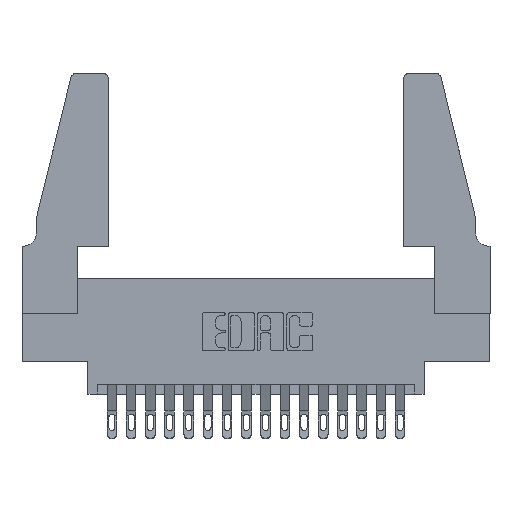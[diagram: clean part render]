
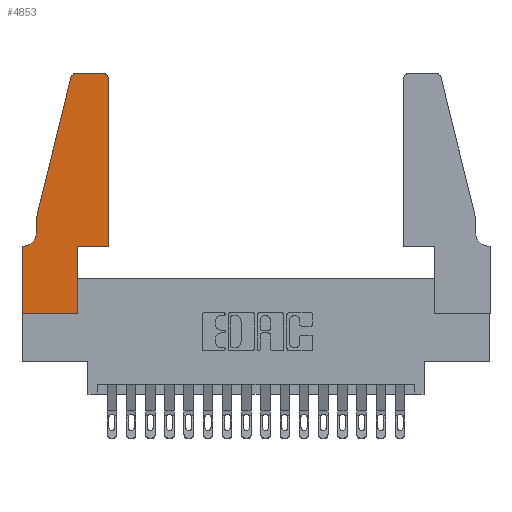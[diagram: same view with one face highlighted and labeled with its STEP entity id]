
A CAD part, top view. The second image highlights one B-rep face of the part: STEP entity #4853.
In plain terms, the highlighted planar face has unit normal (0, 0, 1).
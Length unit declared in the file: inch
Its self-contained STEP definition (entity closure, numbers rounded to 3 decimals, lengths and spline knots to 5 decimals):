
#192 = DIRECTION ( 'NONE',  ( 1., 0., 0. ) ) ;
#594 = EDGE_CURVE ( 'NONE', #18173, #11872, #6268, .T. ) ;
#595 = VECTOR ( 'NONE', #14582, 39.37008 ) ;
#619 = LINE ( 'NONE', #14084, #3350 ) ;
#630 = CARTESIAN_POINT ( 'NONE',  ( 0.0755, 0.5, 0.37 ) ) ;
#766 = LINE ( 'NONE', #17768, #15191 ) ;
#815 = CARTESIAN_POINT ( 'NONE',  ( 0.2605, 1.25, 0.37 ) ) ;
#1052 = VERTEX_POINT ( 'NONE', #14159 ) ;
#1059 = LINE ( 'NONE', #7055, #15020 ) ;
#1093 = DIRECTION ( 'NONE',  ( 0., 1., 0. ) ) ;
#1197 = ORIENTED_EDGE ( 'NONE', *, *, #14014, .T. ) ;
#1435 = EDGE_CURVE ( 'NONE', #11872, #15303, #619, .T. ) ;
#1453 = CARTESIAN_POINT ( 'NONE',  ( 0., 0., 0.37 ) ) ;
#1504 = VERTEX_POINT ( 'NONE', #4140 ) ;
#1822 = EDGE_CURVE ( 'NONE', #4854, #11485, #13237, .T. ) ;
#1848 = EDGE_CURVE ( 'NONE', #17354, #1052, #6470, .T. ) ;
#1901 = VECTOR ( 'NONE', #18646, 39.37008 ) ;
#2020 = EDGE_CURVE ( 'NONE', #1052, #1504, #8303, .T. ) ;
#2126 = DIRECTION ( 'NONE',  ( 0., 0., -1. ) ) ;
#2345 = DIRECTION ( 'NONE',  ( 0., 1., 0. ) ) ;
#2715 = CARTESIAN_POINT ( 'NONE',  ( 0., 0., 0.37 ) ) ;
#3350 = VECTOR ( 'NONE', #1093, 39.37008 ) ;
#4140 = CARTESIAN_POINT ( 'NONE',  ( 0.0755, 0.5, 0.37 ) ) ;
#4509 = CARTESIAN_POINT ( 'NONE',  ( 0., 0.35, 0.37 ) ) ;
#4547 = ORIENTED_EDGE ( 'NONE', *, *, #9464, .T. ) ;
#4673 = DIRECTION ( 'NONE',  ( 1., 0., 0. ) ) ;
#4807 = ORIENTED_EDGE ( 'NONE', *, *, #15778, .T. ) ;
#4853 = ADVANCED_FACE ( 'NONE', ( #9282 ), #7231, .T. ) ;
#4854 = VERTEX_POINT ( 'NONE', #18612 ) ;
#5377 = CARTESIAN_POINT ( 'NONE',  ( 0.2865, 0., 0.37 ) ) ;
#5549 = AXIS2_PLACEMENT_3D ( 'NONE', #10782, #2126, #12234 ) ;
#5876 = VERTEX_POINT ( 'NONE', #14647 ) ;
#5890 = CARTESIAN_POINT ( 'NONE',  ( 0.4205, 1.22, 0.37 ) ) ;
#6268 = LINE ( 'NONE', #1453, #16870 ) ;
#6305 = CARTESIAN_POINT ( 'NONE',  ( 0.4505, 1.22, 0.37 ) ) ;
#6470 = CIRCLE ( 'NONE', #13186, 0.03 ) ;
#6613 = DIRECTION ( 'NONE',  ( 1., 0., 0. ) ) ;
#6715 = ORIENTED_EDGE ( 'NONE', *, *, #1848, .T. ) ;
#6776 = EDGE_LOOP ( 'NONE', ( #15800, #6715, #12855, #10229, #4547, #1197, #4807, #16602, #7133, #7607, #13536, #18490 ) ) ;
#7055 = CARTESIAN_POINT ( 'NONE',  ( 0.0755, 0.35, 0.37 ) ) ;
#7133 = ORIENTED_EDGE ( 'NONE', *, *, #1435, .T. ) ;
#7231 = PLANE ( 'NONE',  #7327 ) ;
#7327 = AXIS2_PLACEMENT_3D ( 'NONE', #4509, #17472, #192 ) ;
#7607 = ORIENTED_EDGE ( 'NONE', *, *, #13905, .T. ) ;
#8265 = VERTEX_POINT ( 'NONE', #9672 ) ;
#8303 = LINE ( 'NONE', #8931, #595 ) ;
#8655 = AXIS2_PLACEMENT_3D ( 'NONE', #5890, #15963, #14579 ) ;
#8827 = VECTOR ( 'NONE', #8945, 39.37008 ) ;
#8931 = CARTESIAN_POINT ( 'NONE',  ( 0.0755, 0.5, 0.37 ) ) ;
#8945 = DIRECTION ( 'NONE',  ( -1., 0., 0. ) ) ;
#9282 = FACE_OUTER_BOUND ( 'NONE', #6776, .T. ) ;
#9390 = CARTESIAN_POINT ( 'NONE',  ( 0.4505, 0.35, 0.37 ) ) ;
#9406 = CARTESIAN_POINT ( 'NONE',  ( 0.4505, 0.35, 0.37 ) ) ;
#9464 = EDGE_CURVE ( 'NONE', #8265, #5876, #14580, .T. ) ;
#9672 = CARTESIAN_POINT ( 'NONE',  ( 0.0755, 0.42, 0.37 ) ) ;
#10229 = ORIENTED_EDGE ( 'NONE', *, *, #10889, .T. ) ;
#10782 = CARTESIAN_POINT ( 'NONE',  ( 0.0055, 0.42, 0.37 ) ) ;
#10889 = EDGE_CURVE ( 'NONE', #1504, #8265, #14748, .T. ) ;
#10925 = VERTEX_POINT ( 'NONE', #13847 ) ;
#11014 = VECTOR ( 'NONE', #6613, 39.37008 ) ;
#11485 = VERTEX_POINT ( 'NONE', #6305 ) ;
#11872 = VERTEX_POINT ( 'NONE', #5377 ) ;
#11950 = EDGE_CURVE ( 'NONE', #13672, #17354, #12441, .T. ) ;
#12234 = DIRECTION ( 'NONE',  ( -1., 0., 0. ) ) ;
#12441 = LINE ( 'NONE', #815, #8827 ) ;
#12554 = CARTESIAN_POINT ( 'NONE',  ( 0.284, 1.25, 0.37 ) ) ;
#12855 = ORIENTED_EDGE ( 'NONE', *, *, #2020, .T. ) ;
#12927 = CIRCLE ( 'NONE', #8655, 0.03 ) ;
#13186 = AXIS2_PLACEMENT_3D ( 'NONE', #14512, #16331, #4673 ) ;
#13237 = LINE ( 'NONE', #9406, #16161 ) ;
#13536 = ORIENTED_EDGE ( 'NONE', *, *, #1822, .T. ) ;
#13672 = VERTEX_POINT ( 'NONE', #16121 ) ;
#13847 = CARTESIAN_POINT ( 'NONE',  ( 0., 0.35, 0.37 ) ) ;
#13905 = EDGE_CURVE ( 'NONE', #15303, #4854, #16621, .T. ) ;
#14014 = EDGE_CURVE ( 'NONE', #5876, #10925, #1059, .T. ) ;
#14084 = CARTESIAN_POINT ( 'NONE',  ( 0.2865, 0.35, 0.37 ) ) ;
#14159 = CARTESIAN_POINT ( 'NONE',  ( 0.25487, 1.22718, 0.37 ) ) ;
#14211 = DIRECTION ( 'NONE',  ( 1., 0., 0. ) ) ;
#14512 = CARTESIAN_POINT ( 'NONE',  ( 0.284, 1.22, 0.37 ) ) ;
#14579 = DIRECTION ( 'NONE',  ( 1., 0., 0. ) ) ;
#14580 = CIRCLE ( 'NONE', #5549, 0.07 ) ;
#14582 = DIRECTION ( 'NONE',  ( -0.239, -0.971, 0. ) ) ;
#14647 = CARTESIAN_POINT ( 'NONE',  ( 0.0055, 0.35, 0.37 ) ) ;
#14748 = LINE ( 'NONE', #630, #1901 ) ;
#15020 = VECTOR ( 'NONE', #16993, 39.37008 ) ;
#15174 = DIRECTION ( 'NONE',  ( 0., -1., 0. ) ) ;
#15191 = VECTOR ( 'NONE', #15174, 39.37008 ) ;
#15303 = VERTEX_POINT ( 'NONE', #15811 ) ;
#15778 = EDGE_CURVE ( 'NONE', #10925, #18173, #766, .T. ) ;
#15800 = ORIENTED_EDGE ( 'NONE', *, *, #11950, .T. ) ;
#15811 = CARTESIAN_POINT ( 'NONE',  ( 0.2865, 0.35, 0.37 ) ) ;
#15963 = DIRECTION ( 'NONE',  ( 0., 0., 1. ) ) ;
#16118 = EDGE_CURVE ( 'NONE', #11485, #13672, #12927, .T. ) ;
#16121 = CARTESIAN_POINT ( 'NONE',  ( 0.4205, 1.25, 0.37 ) ) ;
#16161 = VECTOR ( 'NONE', #2345, 39.37008 ) ;
#16331 = DIRECTION ( 'NONE',  ( 0., 0., 1. ) ) ;
#16602 = ORIENTED_EDGE ( 'NONE', *, *, #594, .T. ) ;
#16621 = LINE ( 'NONE', #9390, #11014 ) ;
#16870 = VECTOR ( 'NONE', #14211, 39.37008 ) ;
#16993 = DIRECTION ( 'NONE',  ( -1., 0., 0. ) ) ;
#17354 = VERTEX_POINT ( 'NONE', #12554 ) ;
#17472 = DIRECTION ( 'NONE',  ( 0., 0., 1. ) ) ;
#17768 = CARTESIAN_POINT ( 'NONE',  ( 0., 0., 0.37 ) ) ;
#18173 = VERTEX_POINT ( 'NONE', #2715 ) ;
#18490 = ORIENTED_EDGE ( 'NONE', *, *, #16118, .T. ) ;
#18612 = CARTESIAN_POINT ( 'NONE',  ( 0.4505, 0.35, 0.37 ) ) ;
#18646 = DIRECTION ( 'NONE',  ( 0., -1., 0. ) ) ;
